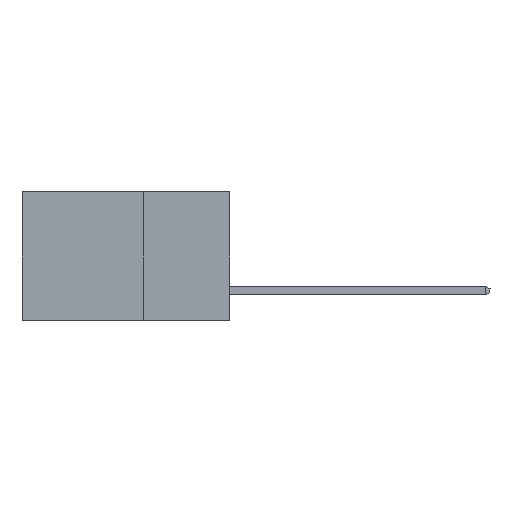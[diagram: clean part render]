
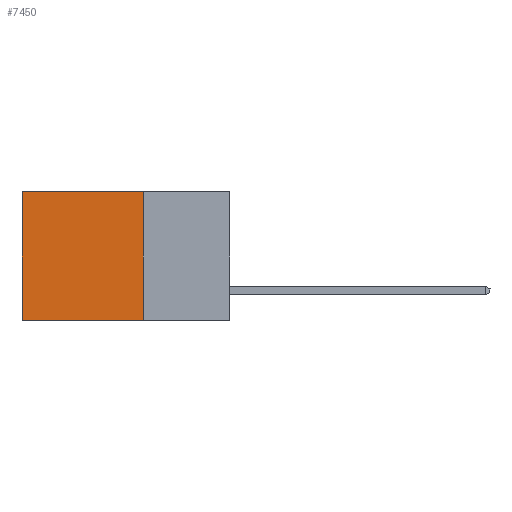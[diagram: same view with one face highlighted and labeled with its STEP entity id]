
A CAD part, left-side view. The second image highlights one B-rep face of the part: STEP entity #7450.
In plain terms, the highlighted planar face has unit normal (-1, 0, 0).
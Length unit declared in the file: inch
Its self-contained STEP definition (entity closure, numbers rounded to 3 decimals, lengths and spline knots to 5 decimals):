
#831 = ORIENTED_EDGE ( 'NONE', *, *, #6268, .T. ) ;
#874 = VECTOR ( 'NONE', #4725, 39.37008 ) ;
#889 = EDGE_LOOP ( 'NONE', ( #831, #6225, #3498, #1321 ) ) ;
#1232 = CARTESIAN_POINT ( 'NONE',  ( 0.2615, 0.25, -0.37 ) ) ;
#1321 = ORIENTED_EDGE ( 'NONE', *, *, #5582, .T. ) ;
#2096 = LINE ( 'NONE', #5986, #9977 ) ;
#2461 = CARTESIAN_POINT ( 'NONE',  ( 0.2615, 0.25, -0.37 ) ) ;
#3258 = CARTESIAN_POINT ( 'NONE',  ( 0.2615, 0.25, -0.37 ) ) ;
#3481 = VECTOR ( 'NONE', #5861, 39.37008 ) ;
#3498 = ORIENTED_EDGE ( 'NONE', *, *, #4384, .F. ) ;
#3862 = CARTESIAN_POINT ( 'NONE',  ( 0.2615, 0.6, -0.37 ) ) ;
#4052 = EDGE_CURVE ( 'NONE', #4686, #11311, #9003, .T. ) ;
#4384 = EDGE_CURVE ( 'NONE', #7648, #4686, #9658, .T. ) ;
#4621 = AXIS2_PLACEMENT_3D ( 'NONE', #3258, #7804, #9678 ) ;
#4686 = VERTEX_POINT ( 'NONE', #9343 ) ;
#4725 = DIRECTION ( 'NONE',  ( 0., 1., 0. ) ) ;
#5582 = EDGE_CURVE ( 'NONE', #7648, #11647, #5736, .T. ) ;
#5736 = LINE ( 'NONE', #10311, #874 ) ;
#5861 = DIRECTION ( 'NONE',  ( 0., 0., -1. ) ) ;
#5986 = CARTESIAN_POINT ( 'NONE',  ( 0.2615, 0.6, -0.37 ) ) ;
#6225 = ORIENTED_EDGE ( 'NONE', *, *, #4052, .F. ) ;
#6268 = EDGE_CURVE ( 'NONE', #11647, #11311, #2096, .T. ) ;
#6770 = DIRECTION ( 'NONE',  ( 0., 0., -1. ) ) ;
#7450 = ADVANCED_FACE ( 'NONE', ( #9614 ), #8642, .F. ) ;
#7648 = VERTEX_POINT ( 'NONE', #11696 ) ;
#7804 = DIRECTION ( 'NONE',  ( 1., 0., 0. ) ) ;
#8642 = PLANE ( 'NONE',  #4621 ) ;
#9003 = LINE ( 'NONE', #2461, #10712 ) ;
#9343 = CARTESIAN_POINT ( 'NONE',  ( 0.2615, 0.25, -0.37 ) ) ;
#9614 = FACE_OUTER_BOUND ( 'NONE', #889, .T. ) ;
#9658 = LINE ( 'NONE', #1232, #3481 ) ;
#9678 = DIRECTION ( 'NONE',  ( 0., 0., -1. ) ) ;
#9893 = CARTESIAN_POINT ( 'NONE',  ( 0.2615, 0.6, 0. ) ) ;
#9977 = VECTOR ( 'NONE', #6770, 39.37008 ) ;
#10311 = CARTESIAN_POINT ( 'NONE',  ( 0.2615, 0.25, 0. ) ) ;
#10712 = VECTOR ( 'NONE', #11876, 39.37008 ) ;
#11311 = VERTEX_POINT ( 'NONE', #3862 ) ;
#11647 = VERTEX_POINT ( 'NONE', #9893 ) ;
#11696 = CARTESIAN_POINT ( 'NONE',  ( 0.2615, 0.25, 0. ) ) ;
#11876 = DIRECTION ( 'NONE',  ( 0., 1., 0. ) ) ;
